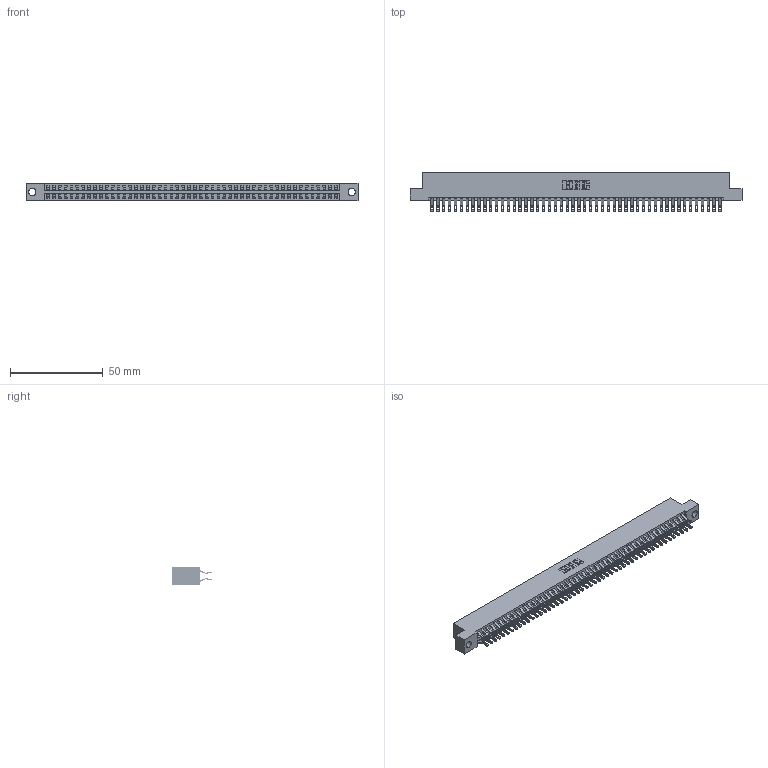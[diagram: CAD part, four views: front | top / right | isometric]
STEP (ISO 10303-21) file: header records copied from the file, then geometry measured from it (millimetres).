
FILE_DESCRIPTION (( 'STEP AP203' ), '1' );
FILE_NAME ('396-100-555-204.STEP', '2018-09-14T07:40:26', ( '' ), ( '' ), 'SwSTEP 2.0', 'SolidWorks 2016', '' );
FILE_SCHEMA (( 'CONFIG_CONTROL_DESIGN' ));
Length unit declared in the file: inch
Products named in the file (3): 346 Part_Flush Mounting Lugs - 0.156 Dia-TH; 345-292-001_555 Tail; 396-100-555-204
Assembly tree (101 placements, depth 2):
  396-100-555-204
    346 Part_Flush Mounting Lugs - 0.156 Dia-TH
    345-292-001_555 Tail  x100
Bounding box: 179.32 x 21.46 x 9.4 mm (x, y, z)
Volume: 17750.6 mm3; surface area: 25372.5 mm2
Topology: 101 solids, 101 shells, 5922 faces, 18629 edges, 12418 vertices
Faces by surface type: plane 3376, cylinder 2546
Entity records: 31883 total; most frequent: CARTESIAN_POINT 5278, ORIENTED_EDGE 5182, DIRECTION 4671, EDGE_CURVE 2591, VECTOR 2239, LINE 2239, VERTEX_POINT 1726, AXIS2_PLACEMENT_3D 1216
